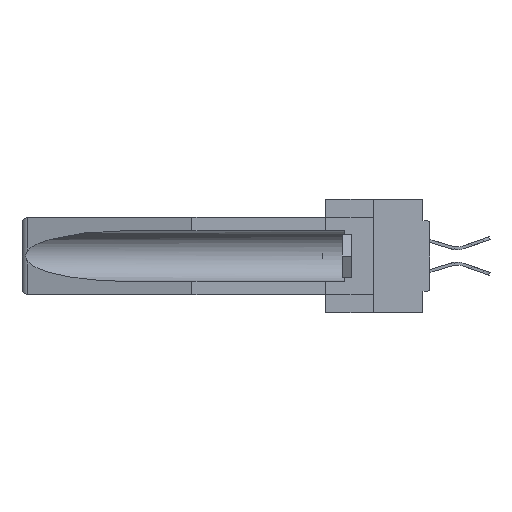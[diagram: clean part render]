
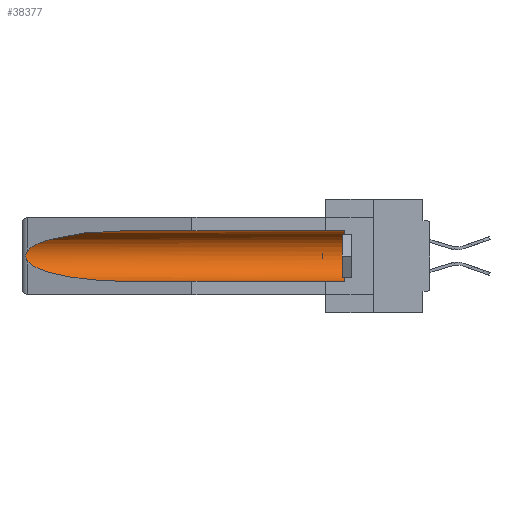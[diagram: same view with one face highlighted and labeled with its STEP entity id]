
A CAD part, left-side view. The second image highlights one B-rep face of the part: STEP entity #38377.
In plain terms, the highlighted cylindrical face has radius 2.857 mm (diameter 5.715 mm), a partial arc.
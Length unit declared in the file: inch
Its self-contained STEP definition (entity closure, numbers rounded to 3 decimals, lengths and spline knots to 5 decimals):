
#312 = FACE_OUTER_BOUND ( 'NONE', #13391, .T. ) ;
#1765 = CARTESIAN_POINT ( 'NONE',  ( 0.2675, 1.53308, -0.17534 ) ) ;
#3331 = EDGE_CURVE ( 'NONE', #32417, #6973, #20236, .T. ) ;
#5313 = DIRECTION ( 'NONE',  ( 0., 1., 0. ) ) ;
#5571 = CARTESIAN_POINT ( 'NONE',  ( 0.2673, 1.53269, -0.17917 ) ) ;
#5782 = EDGE_CURVE ( 'NONE', #12928, #45617, #25146, .T. ) ;
#6704 = CARTESIAN_POINT ( 'NONE',  ( 0.155, 0.126, -0.059 ) ) ;
#6973 = VERTEX_POINT ( 'NONE', #6704 ) ;
#7144 = CARTESIAN_POINT ( 'NONE',  ( 0.155, 1.07973, -0.284 ) ) ;
#7920 = CARTESIAN_POINT ( 'NONE',  ( 0.155, 1.07973, -0.059 ) ) ;
#9075 = ORIENTED_EDGE ( 'NONE', *, *, #3331, .T. ) ;
#10055 = EDGE_CURVE ( 'NONE', #22273, #12928, #14092, .T. ) ;
#11869 = CARTESIAN_POINT ( 'NONE',  ( 0.155, 1.07973, -0.284 ) ) ;
#12384 = CARTESIAN_POINT ( 'NONE',  ( 0.26597, 1.5296, -0.19026 ) ) ;
#12928 = VERTEX_POINT ( 'NONE', #33995 ) ;
#13050 = CARTESIAN_POINT ( 'NONE',  ( 0.26597, 1.52961, -0.15275 ) ) ;
#13391 = EDGE_LOOP ( 'NONE', ( #27304, #20406, #38315, #15877, #9075, #37740 ) ) ;
#14092 =( BOUNDED_CURVE ( )  B_SPLINE_CURVE ( 3, ( #7920, #15258, #45855, #42650 ),
 .UNSPECIFIED., .F., .F. ) 
 B_SPLINE_CURVE_WITH_KNOTS ( ( 4, 4 ),
 ( 4.71239, 6.08839 ),
 .UNSPECIFIED. ) 
 CURVE ( )  GEOMETRIC_REPRESENTATION_ITEM ( )  RATIONAL_B_SPLINE_CURVE ( ( 1., 0.848, 0.848, 1. ) ) 
 REPRESENTATION_ITEM ( '' )  );
#14779 = VECTOR ( 'NONE', #26041, 39.37008 ) ;
#15258 = CARTESIAN_POINT ( 'NONE',  ( 0.21114, 1.30732, -0.059 ) ) ;
#15575 = CARTESIAN_POINT ( 'NONE',  ( 0.155, 0.126, -0.284 ) ) ;
#15877 = ORIENTED_EDGE ( 'NONE', *, *, #36310, .F. ) ;
#20236 = CIRCLE ( 'NONE', #22114, 0.1125 ) ;
#20250 = VECTOR ( 'NONE', #31819, 39.37008 ) ;
#20406 = ORIENTED_EDGE ( 'NONE', *, *, #5782, .T. ) ;
#22114 = AXIS2_PLACEMENT_3D ( 'NONE', #35343, #31195, #23997 ) ;
#22273 = VERTEX_POINT ( 'NONE', #34887 ) ;
#23980 = CARTESIAN_POINT ( 'NONE',  ( 0.155, -0.30754, -0.059 ) ) ;
#23997 = DIRECTION ( 'NONE',  ( 0., 0., 1. ) ) ;
#24601 = CARTESIAN_POINT ( 'NONE',  ( 0.2675, 1.53308, -0.16763 ) ) ;
#25146 = B_SPLINE_CURVE_WITH_KNOTS ( 'NONE', 3,
 ( #47317, #13050, #32282, #43661, #24601, #1765, #5571, #35274, #12384, #39148 ),
 .UNSPECIFIED., .F., .F.,
 ( 4, 2, 2, 2, 4 ),
 ( 0., 0.00029, 0.00058, 0.00087, 0.00117 ),
 .UNSPECIFIED. ) ;
#26041 = DIRECTION ( 'NONE',  ( 0., 1., 0. ) ) ;
#26240 = LINE ( 'NONE', #23980, #20250 ) ;
#27304 = ORIENTED_EDGE ( 'NONE', *, *, #10055, .T. ) ;
#27787 = EDGE_CURVE ( 'NONE', #6973, #22273, #26240, .T. ) ;
#29341 = CARTESIAN_POINT ( 'NONE',  ( 0.21114, 1.30732, -0.284 ) ) ;
#30766 = AXIS2_PLACEMENT_3D ( 'NONE', #39221, #5313, #39710 ) ;
#31195 = DIRECTION ( 'NONE',  ( 0., -1., 0. ) ) ;
#31819 = DIRECTION ( 'NONE',  ( 0., 1., 0. ) ) ;
#31971 = CYLINDRICAL_SURFACE ( 'NONE', #30766, 0.1125 ) ;
#32282 = CARTESIAN_POINT ( 'NONE',  ( 0.26654, 1.53092, -0.15636 ) ) ;
#32417 = VERTEX_POINT ( 'NONE', #15575 ) ;
#33995 = CARTESIAN_POINT ( 'NONE',  ( 0.26537, 1.52718, -0.14972 ) ) ;
#34887 = CARTESIAN_POINT ( 'NONE',  ( 0.155, 1.07973, -0.059 ) ) ;
#35274 = CARTESIAN_POINT ( 'NONE',  ( 0.26655, 1.53094, -0.18657 ) ) ;
#35343 = CARTESIAN_POINT ( 'NONE',  ( 0.155, 0.126, -0.1715 ) ) ;
#35756 =( BOUNDED_CURVE ( )  B_SPLINE_CURVE ( 3, ( #44235, #48070, #29341, #7144 ),
 .UNSPECIFIED., .F., .T. ) 
 B_SPLINE_CURVE_WITH_KNOTS ( ( 4, 4 ),
 ( 0.1948, 1.5708 ),
 .UNSPECIFIED. ) 
 CURVE ( )  GEOMETRIC_REPRESENTATION_ITEM ( )  RATIONAL_B_SPLINE_CURVE ( ( 1., 0.848, 0.848, 1. ) ) 
 REPRESENTATION_ITEM ( '' )  );
#36310 = EDGE_CURVE ( 'NONE', #32417, #40475, #39924, .T. ) ;
#37728 = CARTESIAN_POINT ( 'NONE',  ( 0.155, -0.30754, -0.284 ) ) ;
#37740 = ORIENTED_EDGE ( 'NONE', *, *, #27787, .T. ) ;
#38315 = ORIENTED_EDGE ( 'NONE', *, *, #43946, .T. ) ;
#38377 = ADVANCED_FACE ( 'NONE', ( #312 ), #31971, .F. ) ;
#39148 = CARTESIAN_POINT ( 'NONE',  ( 0.26537, 1.52718, -0.19328 ) ) ;
#39221 = CARTESIAN_POINT ( 'NONE',  ( 0.155, -0.30754, -0.1715 ) ) ;
#39710 = DIRECTION ( 'NONE',  ( 0., 0., 1. ) ) ;
#39924 = LINE ( 'NONE', #37728, #14779 ) ;
#40475 = VERTEX_POINT ( 'NONE', #11869 ) ;
#42650 = CARTESIAN_POINT ( 'NONE',  ( 0.26537, 1.52718, -0.14972 ) ) ;
#43661 = CARTESIAN_POINT ( 'NONE',  ( 0.2673, 1.5327, -0.16383 ) ) ;
#43946 = EDGE_CURVE ( 'NONE', #45617, #40475, #35756, .T. ) ;
#44235 = CARTESIAN_POINT ( 'NONE',  ( 0.26537, 1.52718, -0.19328 ) ) ;
#45617 = VERTEX_POINT ( 'NONE', #48751 ) ;
#45855 = CARTESIAN_POINT ( 'NONE',  ( 0.25451, 1.48313, -0.09465 ) ) ;
#47317 = CARTESIAN_POINT ( 'NONE',  ( 0.26537, 1.52718, -0.14972 ) ) ;
#48070 = CARTESIAN_POINT ( 'NONE',  ( 0.25451, 1.48313, -0.24835 ) ) ;
#48751 = CARTESIAN_POINT ( 'NONE',  ( 0.26537, 1.52718, -0.19328 ) ) ;
